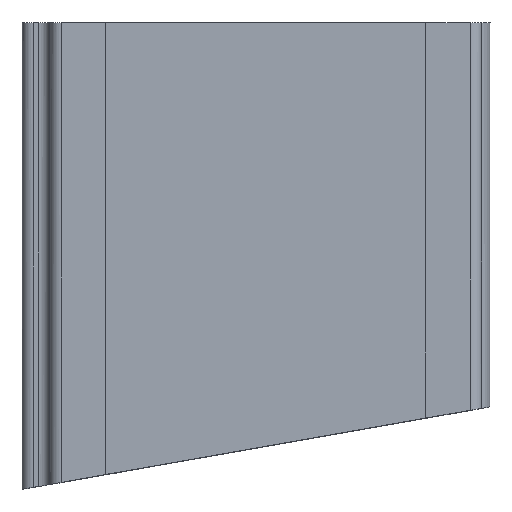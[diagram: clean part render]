
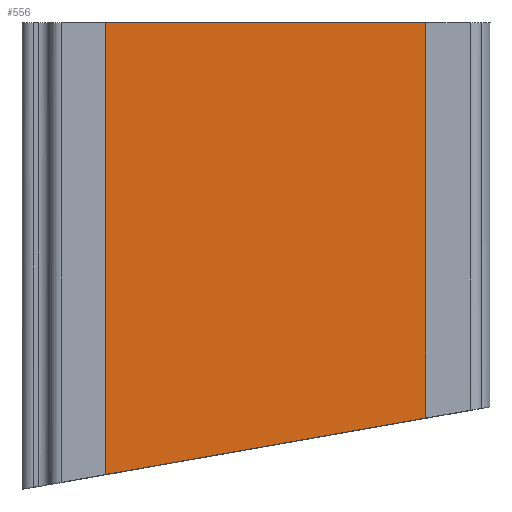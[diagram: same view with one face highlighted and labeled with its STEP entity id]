
A CAD part, top view. The second image highlights one B-rep face of the part: STEP entity #556.
In plain terms, the highlighted planar face has unit normal (0, 0, 1).
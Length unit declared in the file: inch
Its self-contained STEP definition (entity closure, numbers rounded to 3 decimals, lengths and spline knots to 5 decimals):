
#108 = EDGE_CURVE ( 'NONE', #1291, #1317, #1408, .T. ) ;
#110 = CARTESIAN_POINT ( 'NONE',  ( -2.438, -2.2607, 0.4665 ) ) ;
#122 = EDGE_CURVE ( 'NONE', #1291, #1211, #1110, .T. ) ;
#148 = EDGE_CURVE ( 'NONE', #1317, #1335, #1038, .T. ) ;
#162 = CARTESIAN_POINT ( 'NONE',  ( -2.438, 0.2505, 0.4665 ) ) ;
#179 = CARTESIAN_POINT ( 'NONE',  ( -0.66, 0.2505, 0.4665 ) ) ;
#196 = LINE ( 'NONE', #1176, #954 ) ;
#252 = ORIENTED_EDGE ( 'NONE', *, *, #122, .F. ) ;
#261 = ORIENTED_EDGE ( 'NONE', *, *, #108, .T. ) ;
#264 = ORIENTED_EDGE ( 'NONE', *, *, #590, .T. ) ;
#286 = CARTESIAN_POINT ( 'NONE',  ( -0.66, -1.94719, 0.4665 ) ) ;
#341 = VECTOR ( 'NONE', #1275, 39.37008 ) ;
#364 = AXIS2_PLACEMENT_3D ( 'NONE', #1322, #1298, #1294 ) ;
#402 = ORIENTED_EDGE ( 'NONE', *, *, #148, .T. ) ;
#556 = ADVANCED_FACE ( 'NONE', ( #1236 ), #1312, .T. ) ;
#590 = EDGE_CURVE ( 'NONE', #1335, #1211, #196, .T. ) ;
#697 = DIRECTION ( 'NONE',  ( -1., 0., 0. ) ) ;
#786 = CARTESIAN_POINT ( 'NONE',  ( -0.66, 0.2505, 0.4665 ) ) ;
#801 = EDGE_LOOP ( 'NONE', ( #252, #261, #402, #264 ) ) ;
#954 = VECTOR ( 'NONE', #1171, 39.37008 ) ;
#1038 = LINE ( 'NONE', #1146, #341 ) ;
#1078 = VECTOR ( 'NONE', #1334, 39.37008 ) ;
#1110 = LINE ( 'NONE', #786, #1078 ) ;
#1146 = CARTESIAN_POINT ( 'NONE',  ( -2.438, 0.2505, 0.4665 ) ) ;
#1171 = DIRECTION ( 'NONE',  ( 0.985, 0.174, 0. ) ) ;
#1176 = CARTESIAN_POINT ( 'NONE',  ( -2.438, -2.2607, 0.4665 ) ) ;
#1211 = VERTEX_POINT ( 'NONE', #286 ) ;
#1236 = FACE_OUTER_BOUND ( 'NONE', #801, .T. ) ;
#1275 = DIRECTION ( 'NONE',  ( 0., -1., 0. ) ) ;
#1285 = VECTOR ( 'NONE', #697, 39.37008 ) ;
#1291 = VERTEX_POINT ( 'NONE', #179 ) ;
#1294 = DIRECTION ( 'NONE',  ( 1., 0., 0. ) ) ;
#1298 = DIRECTION ( 'NONE',  ( 0., 0., 1. ) ) ;
#1312 = PLANE ( 'NONE',  #364 ) ;
#1317 = VERTEX_POINT ( 'NONE', #162 ) ;
#1322 = CARTESIAN_POINT ( 'NONE',  ( -2.438, 0.2505, 0.4665 ) ) ;
#1334 = DIRECTION ( 'NONE',  ( 0., -1., 0. ) ) ;
#1335 = VERTEX_POINT ( 'NONE', #110 ) ;
#1408 = LINE ( 'NONE', #1510, #1285 ) ;
#1510 = CARTESIAN_POINT ( 'NONE',  ( -0.66, 0.2505, 0.4665 ) ) ;
